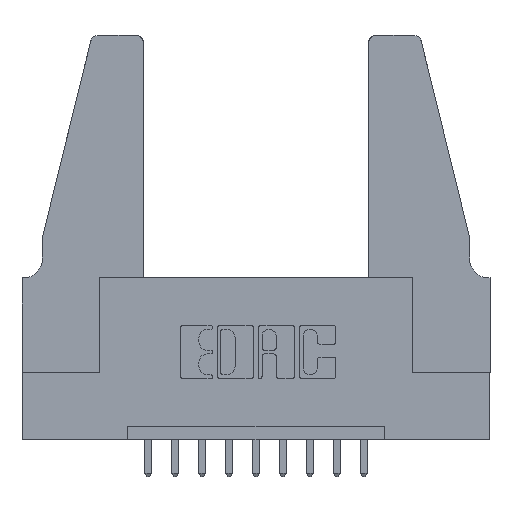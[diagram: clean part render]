
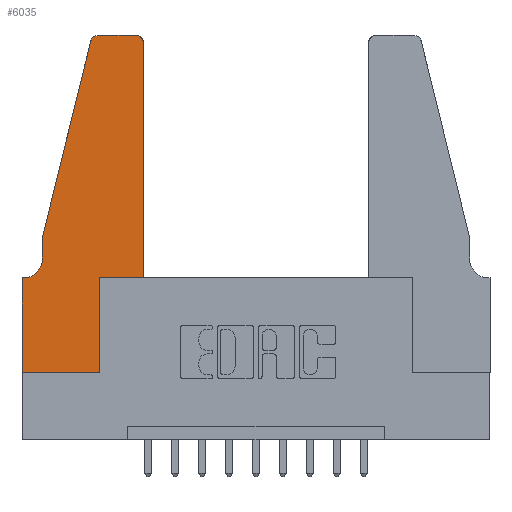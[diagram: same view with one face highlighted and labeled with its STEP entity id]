
A CAD part, top view. The second image highlights one B-rep face of the part: STEP entity #6035.
In plain terms, the highlighted planar face has unit normal (0, 0, 1).
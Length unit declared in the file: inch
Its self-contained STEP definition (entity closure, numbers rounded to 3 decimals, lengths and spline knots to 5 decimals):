
#157 = DIRECTION ( 'NONE',  ( 0., 0., 1. ) ) ;
#170 = CARTESIAN_POINT ( 'NONE',  ( 0.0755, 0.35, 0.37 ) ) ;
#316 = CARTESIAN_POINT ( 'NONE',  ( 0., 0., 0.37 ) ) ;
#621 = CARTESIAN_POINT ( 'NONE',  ( 0.4205, 1.22, 0.37 ) ) ;
#670 = VERTEX_POINT ( 'NONE', #10469 ) ;
#786 = DIRECTION ( 'NONE',  ( 0., 1., 0. ) ) ;
#1015 = FACE_OUTER_BOUND ( 'NONE', #3827, .T. ) ;
#1039 = VECTOR ( 'NONE', #8021, 39.37008 ) ;
#1095 = ORIENTED_EDGE ( 'NONE', *, *, #5923, .T. ) ;
#1167 = ORIENTED_EDGE ( 'NONE', *, *, #12468, .T. ) ;
#1195 = DIRECTION ( 'NONE',  ( 0., -1., 0. ) ) ;
#1250 = CIRCLE ( 'NONE', #4829, 0.07 ) ;
#1282 = DIRECTION ( 'NONE',  ( 0., 0., -1. ) ) ;
#1378 = EDGE_CURVE ( 'NONE', #2029, #10454, #11352, .T. ) ;
#1448 = DIRECTION ( 'NONE',  ( 1., 0., 0. ) ) ;
#1653 = EDGE_CURVE ( 'NONE', #5521, #11598, #6517, .T. ) ;
#2029 = VERTEX_POINT ( 'NONE', #7241 ) ;
#2190 = AXIS2_PLACEMENT_3D ( 'NONE', #2622, #9653, #2489 ) ;
#2329 = DIRECTION ( 'NONE',  ( 1., 0., 0. ) ) ;
#2489 = DIRECTION ( 'NONE',  ( 1., 0., 0. ) ) ;
#2622 = CARTESIAN_POINT ( 'NONE',  ( 0.284, 1.22, 0.37 ) ) ;
#2732 = CARTESIAN_POINT ( 'NONE',  ( 0.4505, 0.35, 0.37 ) ) ;
#2799 = EDGE_CURVE ( 'NONE', #10454, #5784, #7743, .T. ) ;
#3086 = CARTESIAN_POINT ( 'NONE',  ( 0.4505, 0.35, 0.37 ) ) ;
#3135 = CARTESIAN_POINT ( 'NONE',  ( 0.0755, 0.5, 0.37 ) ) ;
#3179 = ORIENTED_EDGE ( 'NONE', *, *, #1378, .T. ) ;
#3339 = CARTESIAN_POINT ( 'NONE',  ( 0.2605, 1.25, 0.37 ) ) ;
#3353 = CARTESIAN_POINT ( 'NONE',  ( 0.284, 1.25, 0.37 ) ) ;
#3422 = CARTESIAN_POINT ( 'NONE',  ( 0.2865, 0.35, 0.37 ) ) ;
#3827 = EDGE_LOOP ( 'NONE', ( #5265, #8354, #3831, #7072, #8774, #1167, #7374, #13365, #1095, #8294, #6111, #3179 ) ) ;
#3831 = ORIENTED_EDGE ( 'NONE', *, *, #12189, .T. ) ;
#3841 = VERTEX_POINT ( 'NONE', #9121 ) ;
#4244 = CARTESIAN_POINT ( 'NONE',  ( 0.0755, 0.5, 0.37 ) ) ;
#4328 = VERTEX_POINT ( 'NONE', #6584 ) ;
#4829 = AXIS2_PLACEMENT_3D ( 'NONE', #11498, #1282, #8541 ) ;
#4831 = CARTESIAN_POINT ( 'NONE',  ( 0.0755, 0.5, 0.37 ) ) ;
#5010 = VECTOR ( 'NONE', #11630, 39.37008 ) ;
#5114 = EDGE_CURVE ( 'NONE', #670, #4328, #8199, .T. ) ;
#5204 = VERTEX_POINT ( 'NONE', #3086 ) ;
#5265 = ORIENTED_EDGE ( 'NONE', *, *, #2799, .T. ) ;
#5521 = VERTEX_POINT ( 'NONE', #4244 ) ;
#5523 = AXIS2_PLACEMENT_3D ( 'NONE', #621, #11166, #8053 ) ;
#5601 = DIRECTION ( 'NONE',  ( 0., 1., 0. ) ) ;
#5784 = VERTEX_POINT ( 'NONE', #3353 ) ;
#5822 = DIRECTION ( 'NONE',  ( -0.239, -0.971, 0. ) ) ;
#5858 = VECTOR ( 'NONE', #13180, 39.37008 ) ;
#5923 = EDGE_CURVE ( 'NONE', #7899, #11831, #8505, .T. ) ;
#6035 = ADVANCED_FACE ( 'NONE', ( #1015 ), #6402, .T. ) ;
#6111 = ORIENTED_EDGE ( 'NONE', *, *, #6477, .T. ) ;
#6402 = PLANE ( 'NONE',  #7611 ) ;
#6451 = CARTESIAN_POINT ( 'NONE',  ( 0., 0.35, 0.37 ) ) ;
#6477 = EDGE_CURVE ( 'NONE', #5204, #2029, #8791, .T. ) ;
#6517 = LINE ( 'NONE', #3135, #9553 ) ;
#6584 = CARTESIAN_POINT ( 'NONE',  ( 0., 0., 0.37 ) ) ;
#6623 = CARTESIAN_POINT ( 'NONE',  ( 0.2865, 0., 0.37 ) ) ;
#7072 = ORIENTED_EDGE ( 'NONE', *, *, #1653, .T. ) ;
#7083 = CARTESIAN_POINT ( 'NONE',  ( 0.0055, 0.35, 0.37 ) ) ;
#7134 = LINE ( 'NONE', #2732, #5858 ) ;
#7150 = CIRCLE ( 'NONE', #2190, 0.03 ) ;
#7181 = EDGE_CURVE ( 'NONE', #4328, #7899, #8622, .T. ) ;
#7241 = CARTESIAN_POINT ( 'NONE',  ( 0.4505, 1.22, 0.37 ) ) ;
#7374 = ORIENTED_EDGE ( 'NONE', *, *, #5114, .T. ) ;
#7550 = EDGE_CURVE ( 'NONE', #5784, #3841, #7150, .T. ) ;
#7611 = AXIS2_PLACEMENT_3D ( 'NONE', #6451, #157, #2329 ) ;
#7743 = LINE ( 'NONE', #3339, #5010 ) ;
#7806 = VECTOR ( 'NONE', #1448, 39.37008 ) ;
#7899 = VERTEX_POINT ( 'NONE', #6623 ) ;
#8021 = DIRECTION ( 'NONE',  ( 0., -1., 0. ) ) ;
#8053 = DIRECTION ( 'NONE',  ( 1., 0., 0. ) ) ;
#8186 = EDGE_CURVE ( 'NONE', #11831, #5204, #7134, .T. ) ;
#8199 = LINE ( 'NONE', #13076, #1039 ) ;
#8256 = VECTOR ( 'NONE', #8338, 39.37008 ) ;
#8294 = ORIENTED_EDGE ( 'NONE', *, *, #8186, .T. ) ;
#8338 = DIRECTION ( 'NONE',  ( -1., 0., 0. ) ) ;
#8354 = ORIENTED_EDGE ( 'NONE', *, *, #7550, .T. ) ;
#8505 = LINE ( 'NONE', #3422, #12060 ) ;
#8541 = DIRECTION ( 'NONE',  ( -1., 0., 0. ) ) ;
#8622 = LINE ( 'NONE', #316, #7806 ) ;
#8774 = ORIENTED_EDGE ( 'NONE', *, *, #13121, .T. ) ;
#8791 = LINE ( 'NONE', #11081, #10079 ) ;
#9121 = CARTESIAN_POINT ( 'NONE',  ( 0.25487, 1.22718, 0.37 ) ) ;
#9553 = VECTOR ( 'NONE', #1195, 39.37008 ) ;
#9653 = DIRECTION ( 'NONE',  ( 0., 0., 1. ) ) ;
#10079 = VECTOR ( 'NONE', #786, 39.37008 ) ;
#10454 = VERTEX_POINT ( 'NONE', #11674 ) ;
#10469 = CARTESIAN_POINT ( 'NONE',  ( 0., 0.35, 0.37 ) ) ;
#11081 = CARTESIAN_POINT ( 'NONE',  ( 0.4505, 0.35, 0.37 ) ) ;
#11165 = VECTOR ( 'NONE', #5822, 39.37008 ) ;
#11166 = DIRECTION ( 'NONE',  ( 0., 0., 1. ) ) ;
#11293 = CARTESIAN_POINT ( 'NONE',  ( 0.0755, 0.42, 0.37 ) ) ;
#11352 = CIRCLE ( 'NONE', #5523, 0.03 ) ;
#11485 = CARTESIAN_POINT ( 'NONE',  ( 0.2865, 0.35, 0.37 ) ) ;
#11498 = CARTESIAN_POINT ( 'NONE',  ( 0.0055, 0.42, 0.37 ) ) ;
#11598 = VERTEX_POINT ( 'NONE', #11293 ) ;
#11630 = DIRECTION ( 'NONE',  ( -1., 0., 0. ) ) ;
#11659 = VERTEX_POINT ( 'NONE', #7083 ) ;
#11674 = CARTESIAN_POINT ( 'NONE',  ( 0.4205, 1.25, 0.37 ) ) ;
#11680 = LINE ( 'NONE', #170, #8256 ) ;
#11831 = VERTEX_POINT ( 'NONE', #11485 ) ;
#12060 = VECTOR ( 'NONE', #5601, 39.37008 ) ;
#12189 = EDGE_CURVE ( 'NONE', #3841, #5521, #12802, .T. ) ;
#12468 = EDGE_CURVE ( 'NONE', #11659, #670, #11680, .T. ) ;
#12802 = LINE ( 'NONE', #4831, #11165 ) ;
#13076 = CARTESIAN_POINT ( 'NONE',  ( 0., 0., 0.37 ) ) ;
#13121 = EDGE_CURVE ( 'NONE', #11598, #11659, #1250, .T. ) ;
#13180 = DIRECTION ( 'NONE',  ( 1., 0., 0. ) ) ;
#13365 = ORIENTED_EDGE ( 'NONE', *, *, #7181, .T. ) ;
